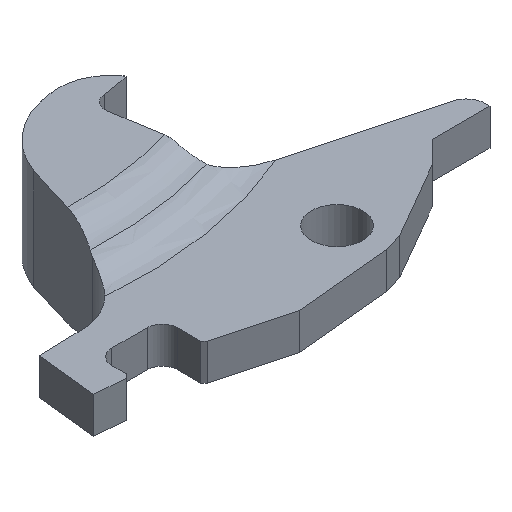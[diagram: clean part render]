
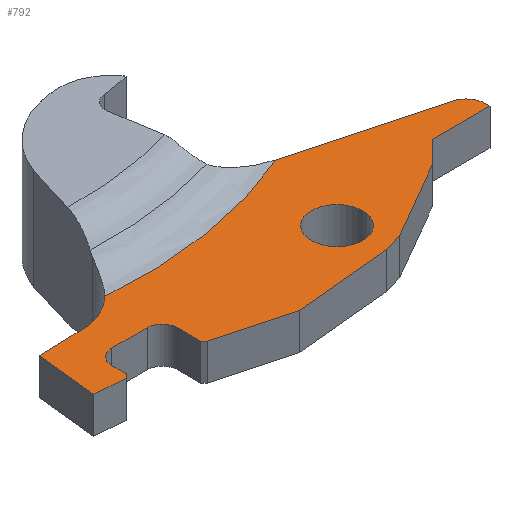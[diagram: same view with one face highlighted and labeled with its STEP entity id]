
A CAD part, isometric view. The second image highlights one B-rep face of the part: STEP entity #792.
In plain terms, the highlighted planar face has unit normal (0, 0, 1).
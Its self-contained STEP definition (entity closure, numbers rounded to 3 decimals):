
#16=FACE_BOUND('',#264,.T.);
#20=PLANE('',#862);
#64=LINE('',#1290,#142);
#69=LINE('',#1326,#147);
#70=LINE('',#1328,#148);
#71=LINE('',#1330,#149);
#72=LINE('',#1332,#150);
#73=LINE('',#1334,#151);
#74=LINE('',#1338,#152);
#75=LINE('',#1342,#153);
#76=LINE('',#1344,#154);
#77=LINE('',#1346,#155);
#78=LINE('',#1348,#156);
#79=LINE('',#1350,#157);
#80=LINE('',#1352,#158);
#81=LINE('',#1354,#159);
#82=LINE('',#1356,#160);
#83=LINE('',#1358,#161);
#142=VECTOR('',#963,10.);
#147=VECTOR('',#984,10.);
#148=VECTOR('',#985,10.);
#149=VECTOR('',#986,10.);
#150=VECTOR('',#987,10.);
#151=VECTOR('',#988,10.);
#152=VECTOR('',#991,10.);
#153=VECTOR('',#994,10.);
#154=VECTOR('',#995,10.);
#155=VECTOR('',#996,10.);
#156=VECTOR('',#997,10.);
#157=VECTOR('',#998,10.);
#158=VECTOR('',#999,10.);
#159=VECTOR('',#1000,10.);
#160=VECTOR('',#1001,10.);
#161=VECTOR('',#1002,10.);
#220=FACE_OUTER_BOUND('',#263,.T.);
#263=EDGE_LOOP('',(#611,#612,#613,#614,#615,#616,#617,#618,#619,#620,#621,
#622,#623,#624,#625,#626,#627,#628,#629,#630,#631));
#264=EDGE_LOOP('',(#632));
#302=CIRCLE('',#847,4.617);
#307=CIRCLE('',#857,32.851);
#311=CIRCLE('',#863,1.176);
#312=CIRCLE('',#864,1.185);
#313=CIRCLE('',#865,1.524);
#314=CIRCLE('',#866,2.);
#350=VERTEX_POINT('',#1199);
#351=VERTEX_POINT('',#1201);
#375=VERTEX_POINT('',#1280);
#376=VERTEX_POINT('',#1289);
#383=VERTEX_POINT('',#1325);
#384=VERTEX_POINT('',#1327);
#385=VERTEX_POINT('',#1329);
#386=VERTEX_POINT('',#1331);
#387=VERTEX_POINT('',#1333);
#388=VERTEX_POINT('',#1335);
#389=VERTEX_POINT('',#1337);
#390=VERTEX_POINT('',#1339);
#391=VERTEX_POINT('',#1341);
#392=VERTEX_POINT('',#1343);
#393=VERTEX_POINT('',#1345);
#394=VERTEX_POINT('',#1347);
#395=VERTEX_POINT('',#1349);
#396=VERTEX_POINT('',#1351);
#397=VERTEX_POINT('',#1353);
#398=VERTEX_POINT('',#1355);
#399=VERTEX_POINT('',#1357);
#400=VERTEX_POINT('',#1360);
#432=EDGE_CURVE('',#350,#351,#302,.T.);
#460=EDGE_CURVE('',#375,#376,#64,.T.);
#467=EDGE_CURVE('',#351,#375,#307,.T.);
#472=EDGE_CURVE('',#383,#350,#69,.T.);
#473=EDGE_CURVE('',#384,#383,#70,.T.);
#474=EDGE_CURVE('',#385,#384,#71,.T.);
#475=EDGE_CURVE('',#386,#385,#72,.T.);
#476=EDGE_CURVE('',#387,#386,#73,.T.);
#477=EDGE_CURVE('',#388,#387,#311,.T.);
#478=EDGE_CURVE('',#389,#388,#74,.T.);
#479=EDGE_CURVE('',#390,#389,#312,.T.);
#480=EDGE_CURVE('',#391,#390,#75,.T.);
#481=EDGE_CURVE('',#392,#391,#76,.T.);
#482=EDGE_CURVE('',#393,#392,#77,.T.);
#483=EDGE_CURVE('',#394,#393,#78,.T.);
#484=EDGE_CURVE('',#395,#394,#79,.T.);
#485=EDGE_CURVE('',#396,#395,#80,.T.);
#486=EDGE_CURVE('',#397,#396,#81,.T.);
#487=EDGE_CURVE('',#398,#397,#82,.T.);
#488=EDGE_CURVE('',#399,#398,#83,.T.);
#489=EDGE_CURVE('',#376,#399,#313,.T.);
#490=EDGE_CURVE('',#400,#400,#314,.T.);
#611=ORIENTED_EDGE('',*,*,#467,.F.);
#612=ORIENTED_EDGE('',*,*,#432,.F.);
#613=ORIENTED_EDGE('',*,*,#472,.F.);
#614=ORIENTED_EDGE('',*,*,#473,.F.);
#615=ORIENTED_EDGE('',*,*,#474,.F.);
#616=ORIENTED_EDGE('',*,*,#475,.F.);
#617=ORIENTED_EDGE('',*,*,#476,.F.);
#618=ORIENTED_EDGE('',*,*,#477,.F.);
#619=ORIENTED_EDGE('',*,*,#478,.F.);
#620=ORIENTED_EDGE('',*,*,#479,.F.);
#621=ORIENTED_EDGE('',*,*,#480,.F.);
#622=ORIENTED_EDGE('',*,*,#481,.F.);
#623=ORIENTED_EDGE('',*,*,#482,.F.);
#624=ORIENTED_EDGE('',*,*,#483,.F.);
#625=ORIENTED_EDGE('',*,*,#484,.F.);
#626=ORIENTED_EDGE('',*,*,#485,.F.);
#627=ORIENTED_EDGE('',*,*,#486,.F.);
#628=ORIENTED_EDGE('',*,*,#487,.F.);
#629=ORIENTED_EDGE('',*,*,#488,.F.);
#630=ORIENTED_EDGE('',*,*,#489,.F.);
#631=ORIENTED_EDGE('',*,*,#460,.F.);
#632=ORIENTED_EDGE('',*,*,#490,.F.);
#792=ADVANCED_FACE('',(#220,#16),#20,.T.);
#847=AXIS2_PLACEMENT_3D('',#1202,#928,#929);
#857=AXIS2_PLACEMENT_3D('',#1313,#972,#973);
#862=AXIS2_PLACEMENT_3D('',#1324,#982,#983);
#863=AXIS2_PLACEMENT_3D('',#1336,#989,#990);
#864=AXIS2_PLACEMENT_3D('',#1340,#992,#993);
#865=AXIS2_PLACEMENT_3D('',#1359,#1003,#1004);
#866=AXIS2_PLACEMENT_3D('',#1361,#1005,#1006);
#928=DIRECTION('center_axis',(0.,0.,1.));
#929=DIRECTION('ref_axis',(0.036,0.999,0.));
#963=DIRECTION('',(0.966,-0.259,0.));
#972=DIRECTION('center_axis',(0.,0.,1.));
#973=DIRECTION('ref_axis',(0.132,-0.991,0.));
#982=DIRECTION('center_axis',(0.,0.,1.));
#983=DIRECTION('ref_axis',(1.,0.,0.));
#984=DIRECTION('',(1.,0.025,0.));
#985=DIRECTION('',(0.102,0.995,0.));
#986=DIRECTION('',(-0.998,0.07,0.));
#987=DIRECTION('',(-0.707,-0.707,0.));
#988=DIRECTION('',(0.,-1.,0.));
#989=DIRECTION('center_axis',(0.,0.,1.));
#990=DIRECTION('ref_axis',(0.,-1.,0.));
#991=DIRECTION('',(-1.,0.,0.));
#992=DIRECTION('center_axis',(0.,0.,1.));
#993=DIRECTION('ref_axis',(-1.,-0.021,0.));
#994=DIRECTION('',(0.,1.,0.));
#995=DIRECTION('',(-0.707,0.707,0.));
#996=DIRECTION('',(-0.966,0.259,0.));
#997=DIRECTION('',(-0.996,-0.093,0.));
#998=DIRECTION('',(-0.953,-0.304,0.));
#999=DIRECTION('',(-0.866,-0.5,0.));
#1000=DIRECTION('',(-0.707,-0.707,0.));
#1001=DIRECTION('',(-1.,0.,0.));
#1002=DIRECTION('',(0.,-1.,0.));
#1003=DIRECTION('center_axis',(0.,0.,-1.));
#1004=DIRECTION('ref_axis',(1.,0.,0.));
#1005=DIRECTION('center_axis',(0.,0.,1.));
#1006=DIRECTION('ref_axis',(-1.,0.,0.));
#1199=CARTESIAN_POINT('',(-18.838,10.189,8.322));
#1201=CARTESIAN_POINT('',(-15.407,11.537,8.322));
#1202=CARTESIAN_POINT('Origin',(-18.67,14.802,8.322));
#1280=CARTESIAN_POINT('',(0.419,14.074,8.322));
#1289=CARTESIAN_POINT('',(11.197,11.187,8.322));
#1290=CARTESIAN_POINT('',(3.882,13.147,8.322));
#1313=CARTESIAN_POINT('Origin',(-12.538,44.262,8.322));
#1324=CARTESIAN_POINT('Origin',(-5.049,9.074,8.322));
#1325=CARTESIAN_POINT('',(-21.94,10.111,8.322));
#1326=CARTESIAN_POINT('',(-11.962,10.362,8.322));
#1327=CARTESIAN_POINT('',(-22.424,5.38,8.322));
#1328=CARTESIAN_POINT('',(-21.906,10.452,8.322));
#1329=CARTESIAN_POINT('',(-20.077,5.215,8.322));
#1330=CARTESIAN_POINT('',(-13.907,4.784,8.322));
#1331=CARTESIAN_POINT('',(-19.779,5.513,8.322));
#1332=CARTESIAN_POINT('',(-15.355,9.937,8.322));
#1333=CARTESIAN_POINT('',(-19.779,6.621,8.322));
#1334=CARTESIAN_POINT('',(-19.779,7.293,8.322));
#1335=CARTESIAN_POINT('',(-18.603,7.799,8.322));
#1336=CARTESIAN_POINT('Origin',(-18.603,6.622,8.322));
#1337=CARTESIAN_POINT('',(-15.86,7.799,8.322));
#1338=CARTESIAN_POINT('',(-11.826,7.799,8.322));
#1339=CARTESIAN_POINT('',(-14.699,6.639,8.322));
#1340=CARTESIAN_POINT('Origin',(-15.885,6.613,8.322));
#1341=CARTESIAN_POINT('',(-14.699,4.809,8.322));
#1342=CARTESIAN_POINT('',(-14.699,7.856,8.322));
#1343=CARTESIAN_POINT('',(-14.449,4.559,8.322));
#1344=CARTESIAN_POINT('',(-13.353,3.463,8.322));
#1345=CARTESIAN_POINT('',(-8.815,3.049,8.322));
#1346=CARTESIAN_POINT('',(-10.628,3.535,8.322));
#1347=CARTESIAN_POINT('',(-1.313,3.75,8.322));
#1348=CARTESIAN_POINT('',(-6.669,3.249,8.322));
#1349=CARTESIAN_POINT('',(0.134,4.211,8.322));
#1350=CARTESIAN_POINT('',(-2.239,3.455,8.322));
#1351=CARTESIAN_POINT('',(6.129,7.672,8.322));
#1352=CARTESIAN_POINT('',(-0.757,3.697,8.322));
#1353=CARTESIAN_POINT('',(7.846,9.389,8.322));
#1354=CARTESIAN_POINT('',(3.685,5.228,8.322));
#1355=CARTESIAN_POINT('',(12.326,9.389,8.322));
#1356=CARTESIAN_POINT('',(1.399,9.389,8.322));
#1357=CARTESIAN_POINT('',(12.326,9.715,8.322));
#1358=CARTESIAN_POINT('',(12.326,9.232,8.322));
#1359=CARTESIAN_POINT('Origin',(10.802,9.715,8.322));
#1360=CARTESIAN_POINT('',(0.356,7.291,8.322));
#1361=CARTESIAN_POINT('Origin',(-1.644,7.291,8.322));
